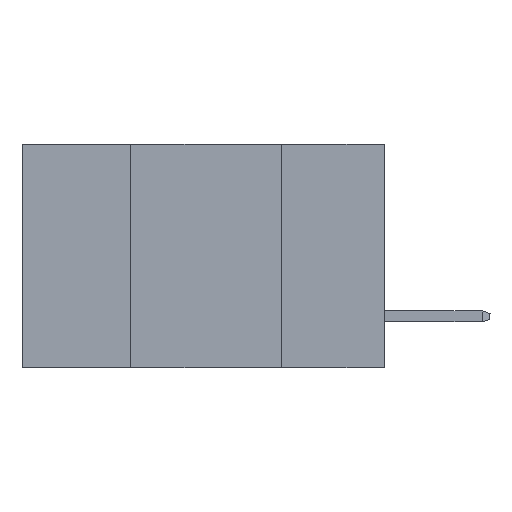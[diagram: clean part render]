
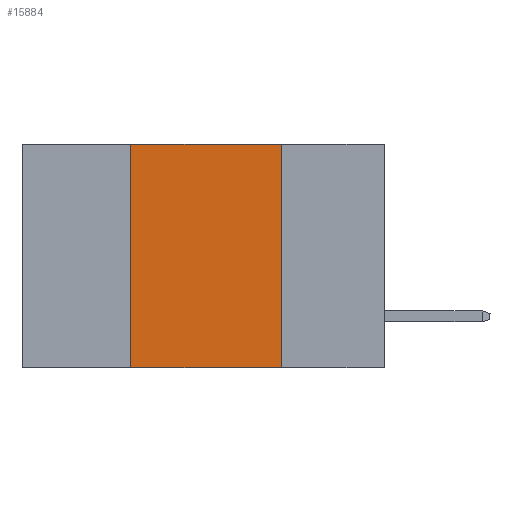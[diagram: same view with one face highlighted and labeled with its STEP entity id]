
A CAD part, left-side view. The second image highlights one B-rep face of the part: STEP entity #15884.
In plain terms, the highlighted planar face has unit normal (-1, 0, 0).
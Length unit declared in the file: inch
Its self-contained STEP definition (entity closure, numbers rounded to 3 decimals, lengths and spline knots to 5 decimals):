
#101 = DIRECTION ( 'NONE',  ( 0., 0., 1. ) ) ;
#892 = LINE ( 'NONE', #7287, #16501 ) ;
#1558 = EDGE_CURVE ( 'NONE', #6294, #4892, #892, .T. ) ;
#2121 = DIRECTION ( 'NONE',  ( 0., -1., 0. ) ) ;
#2714 = FACE_OUTER_BOUND ( 'NONE', #18699, .T. ) ;
#3381 = AXIS2_PLACEMENT_3D ( 'NONE', #12391, #17190, #4092 ) ;
#4036 = ORIENTED_EDGE ( 'NONE', *, *, #6481, .F. ) ;
#4092 = DIRECTION ( 'NONE',  ( 0., 0., -1. ) ) ;
#4302 = ORIENTED_EDGE ( 'NONE', *, *, #20111, .F. ) ;
#4892 = VERTEX_POINT ( 'NONE', #5768 ) ;
#5768 = CARTESIAN_POINT ( 'NONE',  ( 0., 0.17, -0.37 ) ) ;
#5984 = VERTEX_POINT ( 'NONE', #17207 ) ;
#6294 = VERTEX_POINT ( 'NONE', #9168 ) ;
#6481 = EDGE_CURVE ( 'NONE', #15305, #5984, #9900, .T. ) ;
#7057 = ORIENTED_EDGE ( 'NONE', *, *, #1558, .F. ) ;
#7287 = CARTESIAN_POINT ( 'NONE',  ( 0., 0.17, -0.37 ) ) ;
#8366 = CARTESIAN_POINT ( 'NONE',  ( 0., 0.42, -0.37 ) ) ;
#9168 = CARTESIAN_POINT ( 'NONE',  ( 0., 0.17, 0. ) ) ;
#9900 = LINE ( 'NONE', #19400, #12196 ) ;
#12196 = VECTOR ( 'NONE', #101, 39.37008 ) ;
#12391 = CARTESIAN_POINT ( 'NONE',  ( 0., 0.6, 0. ) ) ;
#12418 = DIRECTION ( 'NONE',  ( 0., -1., 0. ) ) ;
#13395 = CARTESIAN_POINT ( 'NONE',  ( 0., 0.6, -0.37 ) ) ;
#13697 = CARTESIAN_POINT ( 'NONE',  ( 0., 0.6, 0. ) ) ;
#15305 = VERTEX_POINT ( 'NONE', #8366 ) ;
#15884 = ADVANCED_FACE ( 'NONE', ( #2714 ), #20085, .F. ) ;
#16243 = VECTOR ( 'NONE', #12418, 39.37008 ) ;
#16501 = VECTOR ( 'NONE', #20427, 39.37008 ) ;
#17190 = DIRECTION ( 'NONE',  ( 1., 0., 0. ) ) ;
#17207 = CARTESIAN_POINT ( 'NONE',  ( 0., 0.42, 0. ) ) ;
#17219 = LINE ( 'NONE', #13697, #16243 ) ;
#17222 = ORIENTED_EDGE ( 'NONE', *, *, #19568, .T. ) ;
#18699 = EDGE_LOOP ( 'NONE', ( #7057, #4302, #4036, #17222 ) ) ;
#18975 = VECTOR ( 'NONE', #2121, 39.37008 ) ;
#19400 = CARTESIAN_POINT ( 'NONE',  ( 0., 0.42, -0.37 ) ) ;
#19568 = EDGE_CURVE ( 'NONE', #15305, #4892, #19720, .T. ) ;
#19720 = LINE ( 'NONE', #13395, #18975 ) ;
#20085 = PLANE ( 'NONE',  #3381 ) ;
#20111 = EDGE_CURVE ( 'NONE', #5984, #6294, #17219, .T. ) ;
#20427 = DIRECTION ( 'NONE',  ( 0., 0., -1. ) ) ;
